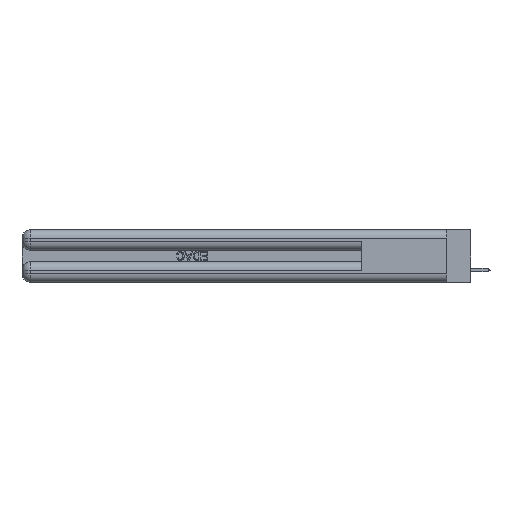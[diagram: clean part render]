
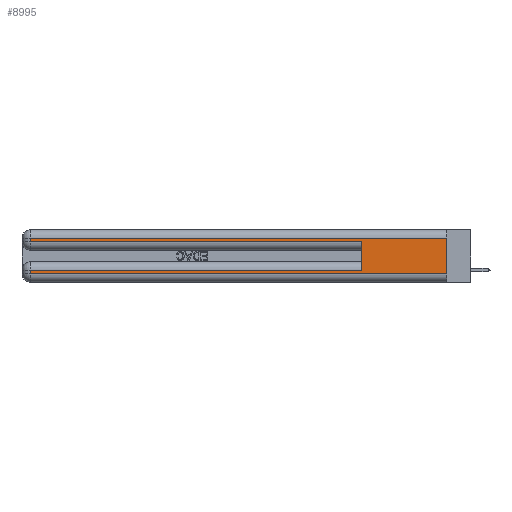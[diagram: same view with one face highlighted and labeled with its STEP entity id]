
A CAD part, left-side view. The second image highlights one B-rep face of the part: STEP entity #8995.
In plain terms, the highlighted planar face has unit normal (-1, 0, 0).
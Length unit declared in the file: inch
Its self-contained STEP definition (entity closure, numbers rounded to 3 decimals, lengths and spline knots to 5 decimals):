
#1239 = EDGE_CURVE ( 'NONE', #41836, #15587, #13433, .T. ) ;
#1346 = ORIENTED_EDGE ( 'NONE', *, *, #23517, .F. ) ;
#2580 = ORIENTED_EDGE ( 'NONE', *, *, #16269, .T. ) ;
#2980 = CARTESIAN_POINT ( 'NONE',  ( 0., 0.6, 0.085 ) ) ;
#4479 = LINE ( 'NONE', #16626, #18487 ) ;
#5229 = CARTESIAN_POINT ( 'NONE',  ( 0., 0.6, 0.145 ) ) ;
#5774 = CARTESIAN_POINT ( 'NONE',  ( 0., 2.94, 0.37 ) ) ;
#6309 = DIRECTION ( 'NONE',  ( 0., 1., 0. ) ) ;
#7097 = EDGE_CURVE ( 'NONE', #33723, #14604, #15129, .T. ) ;
#8995 = ADVANCED_FACE ( 'NONE', ( #20135 ), #32851, .F. ) ;
#9058 = LINE ( 'NONE', #10881, #23605 ) ;
#9319 = DIRECTION ( 'NONE',  ( 0., 0., -1. ) ) ;
#9728 = CARTESIAN_POINT ( 'NONE',  ( 0., 2.94, 0.085 ) ) ;
#10058 = CARTESIAN_POINT ( 'NONE',  ( 0., 2.94, 0.285 ) ) ;
#10307 = CARTESIAN_POINT ( 'NONE',  ( 0., 0., 0.06 ) ) ;
#10421 = AXIS2_PLACEMENT_3D ( 'NONE', #39121, #35910, #9319 ) ;
#10881 = CARTESIAN_POINT ( 'NONE',  ( 0., 0., 0.285 ) ) ;
#11690 = ORIENTED_EDGE ( 'NONE', *, *, #20845, .T. ) ;
#11784 = ORIENTED_EDGE ( 'NONE', *, *, #40329, .T. ) ;
#12785 = CARTESIAN_POINT ( 'NONE',  ( 0., 0., 0.06 ) ) ;
#13433 = LINE ( 'NONE', #5774, #19682 ) ;
#13827 = VERTEX_POINT ( 'NONE', #30776 ) ;
#14177 = VECTOR ( 'NONE', #29896, 39.37008 ) ;
#14604 = VERTEX_POINT ( 'NONE', #10058 ) ;
#14999 = ORIENTED_EDGE ( 'NONE', *, *, #23822, .F. ) ;
#15129 = LINE ( 'NONE', #23764, #38525 ) ;
#15341 = VERTEX_POINT ( 'NONE', #2980 ) ;
#15587 = VERTEX_POINT ( 'NONE', #18367 ) ;
#16269 = EDGE_CURVE ( 'NONE', #14604, #28418, #9058, .T. ) ;
#16626 = CARTESIAN_POINT ( 'NONE',  ( 0., 0., 0.085 ) ) ;
#18367 = CARTESIAN_POINT ( 'NONE',  ( 0., 2.94, 0.06 ) ) ;
#18487 = VECTOR ( 'NONE', #6309, 39.37008 ) ;
#18649 = VECTOR ( 'NONE', #35749, 39.37008 ) ;
#19682 = VECTOR ( 'NONE', #21447, 39.37008 ) ;
#20135 = FACE_OUTER_BOUND ( 'NONE', #22668, .T. ) ;
#20178 = LINE ( 'NONE', #12785, #18649 ) ;
#20423 = LINE ( 'NONE', #39504, #14177 ) ;
#20845 = EDGE_CURVE ( 'NONE', #15587, #27635, #20178, .T. ) ;
#20973 = LINE ( 'NONE', #33996, #41771 ) ;
#21447 = DIRECTION ( 'NONE',  ( 0., 0., -1. ) ) ;
#22018 = CARTESIAN_POINT ( 'NONE',  ( 0., 2.94, 0.31 ) ) ;
#22668 = EDGE_LOOP ( 'NONE', ( #14999, #11784, #29923, #2580, #1346, #25338, #27869, #11690 ) ) ;
#23517 = EDGE_CURVE ( 'NONE', #15341, #28418, #33966, .T. ) ;
#23605 = VECTOR ( 'NONE', #34833, 39.37008 ) ;
#23764 = CARTESIAN_POINT ( 'NONE',  ( 0., 2.94, 0.37 ) ) ;
#23822 = EDGE_CURVE ( 'NONE', #13827, #27635, #20423, .T. ) ;
#25075 = CARTESIAN_POINT ( 'NONE',  ( 0., 0.6, 0.285 ) ) ;
#25338 = ORIENTED_EDGE ( 'NONE', *, *, #26928, .T. ) ;
#26928 = EDGE_CURVE ( 'NONE', #15341, #41836, #4479, .T. ) ;
#27635 = VERTEX_POINT ( 'NONE', #10307 ) ;
#27738 = VECTOR ( 'NONE', #41249, 39.37008 ) ;
#27869 = ORIENTED_EDGE ( 'NONE', *, *, #1239, .T. ) ;
#28418 = VERTEX_POINT ( 'NONE', #25075 ) ;
#29896 = DIRECTION ( 'NONE',  ( 0., 0., -1. ) ) ;
#29923 = ORIENTED_EDGE ( 'NONE', *, *, #7097, .T. ) ;
#30776 = CARTESIAN_POINT ( 'NONE',  ( 0., 0., 0.31 ) ) ;
#32851 = PLANE ( 'NONE',  #10421 ) ;
#33723 = VERTEX_POINT ( 'NONE', #22018 ) ;
#33966 = LINE ( 'NONE', #5229, #27738 ) ;
#33996 = CARTESIAN_POINT ( 'NONE',  ( 0., 0., 0.31 ) ) ;
#34833 = DIRECTION ( 'NONE',  ( 0., -1., 0. ) ) ;
#35749 = DIRECTION ( 'NONE',  ( 0., -1., 0. ) ) ;
#35910 = DIRECTION ( 'NONE',  ( 1., 0., 0. ) ) ;
#37049 = DIRECTION ( 'NONE',  ( 0., 1., 0. ) ) ;
#38525 = VECTOR ( 'NONE', #40503, 39.37008 ) ;
#39121 = CARTESIAN_POINT ( 'NONE',  ( 0., 0., 0.37 ) ) ;
#39504 = CARTESIAN_POINT ( 'NONE',  ( 0., 0., 0.37 ) ) ;
#40329 = EDGE_CURVE ( 'NONE', #13827, #33723, #20973, .T. ) ;
#40503 = DIRECTION ( 'NONE',  ( 0., 0., -1. ) ) ;
#41249 = DIRECTION ( 'NONE',  ( 0., 0., 1. ) ) ;
#41771 = VECTOR ( 'NONE', #37049, 39.37008 ) ;
#41836 = VERTEX_POINT ( 'NONE', #9728 ) ;
